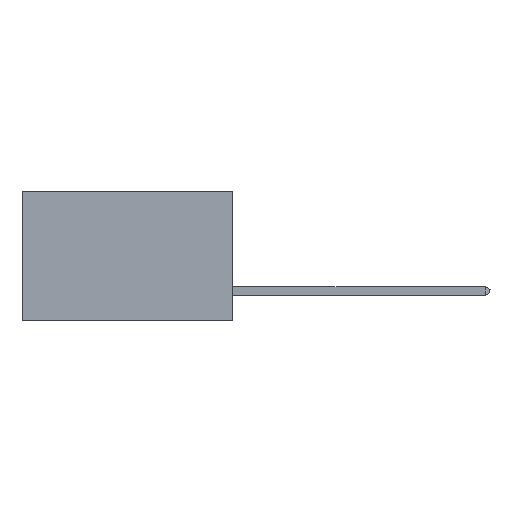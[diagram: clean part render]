
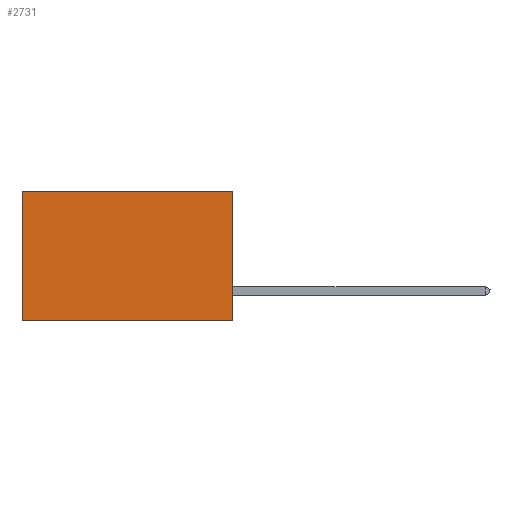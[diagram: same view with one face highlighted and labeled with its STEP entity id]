
A CAD part, left-side view. The second image highlights one B-rep face of the part: STEP entity #2731.
In plain terms, the highlighted planar face has unit normal (-1, 0, 0).
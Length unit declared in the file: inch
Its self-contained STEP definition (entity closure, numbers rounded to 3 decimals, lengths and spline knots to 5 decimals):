
#180 = VERTEX_POINT ( 'NONE', #14733 ) ;
#2684 = VECTOR ( 'NONE', #10186, 39.37008 ) ;
#2731 = ADVANCED_FACE ( 'NONE', ( #9594 ), #5271, .F. ) ;
#2877 = DIRECTION ( 'NONE',  ( 0., 0., -1. ) ) ;
#2887 = LINE ( 'NONE', #25677, #22090 ) ;
#2937 = CARTESIAN_POINT ( 'NONE',  ( 0.2875, 0.6, 0. ) ) ;
#3847 = ORIENTED_EDGE ( 'NONE', *, *, #8330, .F. ) ;
#5271 = PLANE ( 'NONE',  #7904 ) ;
#7260 = ORIENTED_EDGE ( 'NONE', *, *, #22819, .F. ) ;
#7904 = AXIS2_PLACEMENT_3D ( 'NONE', #24506, #10130, #10553 ) ;
#8035 = CARTESIAN_POINT ( 'NONE',  ( 0.2875, 0.6, -0.37 ) ) ;
#8330 = EDGE_CURVE ( 'NONE', #21114, #21241, #14336, .T. ) ;
#9594 = FACE_OUTER_BOUND ( 'NONE', #19198, .T. ) ;
#10110 = EDGE_CURVE ( 'NONE', #180, #17294, #18519, .T. ) ;
#10130 = DIRECTION ( 'NONE',  ( 1., 0., 0. ) ) ;
#10186 = DIRECTION ( 'NONE',  ( 0., 1., 0. ) ) ;
#10251 = CARTESIAN_POINT ( 'NONE',  ( 0.2875, 0., -0.37 ) ) ;
#10553 = DIRECTION ( 'NONE',  ( 0., 0., -1. ) ) ;
#12822 = VECTOR ( 'NONE', #2877, 39.37008 ) ;
#14336 = LINE ( 'NONE', #22354, #12822 ) ;
#14388 = LINE ( 'NONE', #15442, #2684 ) ;
#14733 = CARTESIAN_POINT ( 'NONE',  ( 0.2875, 0.6, 0. ) ) ;
#14780 = VECTOR ( 'NONE', #29483, 39.37008 ) ;
#15442 = CARTESIAN_POINT ( 'NONE',  ( 0.2875, 0., -0.37 ) ) ;
#16124 = ORIENTED_EDGE ( 'NONE', *, *, #10110, .T. ) ;
#16428 = DIRECTION ( 'NONE',  ( 0., 1., 0. ) ) ;
#17294 = VERTEX_POINT ( 'NONE', #8035 ) ;
#18519 = LINE ( 'NONE', #2937, #14780 ) ;
#19198 = EDGE_LOOP ( 'NONE', ( #16124, #7260, #3847, #30695 ) ) ;
#21114 = VERTEX_POINT ( 'NONE', #21743 ) ;
#21241 = VERTEX_POINT ( 'NONE', #10251 ) ;
#21743 = CARTESIAN_POINT ( 'NONE',  ( 0.2875, 0., 0. ) ) ;
#22090 = VECTOR ( 'NONE', #16428, 39.37008 ) ;
#22354 = CARTESIAN_POINT ( 'NONE',  ( 0.2875, 0., 0. ) ) ;
#22819 = EDGE_CURVE ( 'NONE', #21241, #17294, #14388, .T. ) ;
#24506 = CARTESIAN_POINT ( 'NONE',  ( 0.2875, 0., 0. ) ) ;
#25677 = CARTESIAN_POINT ( 'NONE',  ( 0.2875, 0., 0. ) ) ;
#25804 = EDGE_CURVE ( 'NONE', #21114, #180, #2887, .T. ) ;
#29483 = DIRECTION ( 'NONE',  ( 0., 0., -1. ) ) ;
#30695 = ORIENTED_EDGE ( 'NONE', *, *, #25804, .T. ) ;
